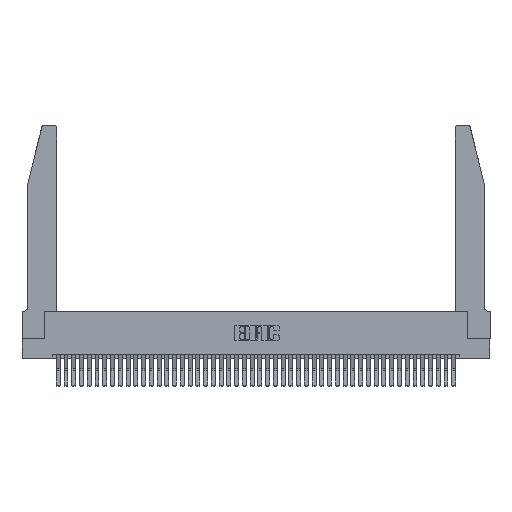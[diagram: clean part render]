
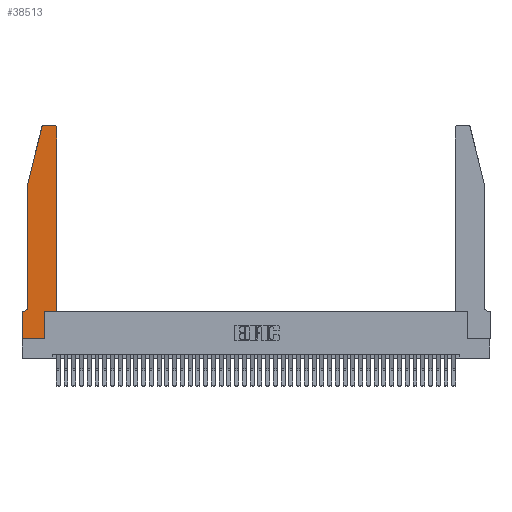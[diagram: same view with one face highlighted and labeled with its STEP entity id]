
A CAD part, top view. The second image highlights one B-rep face of the part: STEP entity #38513.
In plain terms, the highlighted planar face has unit normal (0, 0, 1).
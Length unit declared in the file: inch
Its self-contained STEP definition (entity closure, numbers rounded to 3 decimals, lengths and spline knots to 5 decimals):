
#697 = DIRECTION ( 'NONE',  ( 0., 1., 0. ) ) ;
#743 = VECTOR ( 'NONE', #3688, 39.37008 ) ;
#1118 = VECTOR ( 'NONE', #37977, 39.37008 ) ;
#1593 = CARTESIAN_POINT ( 'NONE',  ( 0., 0., 0.37 ) ) ;
#2560 = EDGE_CURVE ( 'NONE', #4045, #33339, #9989, .T. ) ;
#3688 = DIRECTION ( 'NONE',  ( -1., 0., 0. ) ) ;
#3888 = DIRECTION ( 'NONE',  ( 0., -1., 0. ) ) ;
#4045 = VERTEX_POINT ( 'NONE', #23233 ) ;
#4098 = VERTEX_POINT ( 'NONE', #26815 ) ;
#5146 = CIRCLE ( 'NONE', #24599, 0.03 ) ;
#5670 = CARTESIAN_POINT ( 'NONE',  ( 0.284, 2.72, 0.37 ) ) ;
#6162 = VERTEX_POINT ( 'NONE', #10857 ) ;
#6291 = CARTESIAN_POINT ( 'NONE',  ( 0.0755, 2., 0.37 ) ) ;
#7109 = DIRECTION ( 'NONE',  ( 0., 0., 1. ) ) ;
#8375 = VERTEX_POINT ( 'NONE', #39260 ) ;
#9040 = ORIENTED_EDGE ( 'NONE', *, *, #27470, .T. ) ;
#9112 = DIRECTION ( 'NONE',  ( 1., 0., 0. ) ) ;
#9331 = VERTEX_POINT ( 'NONE', #37391 ) ;
#9704 = DIRECTION ( 'NONE',  ( -0.239, -0.971, 0. ) ) ;
#9774 = ORIENTED_EDGE ( 'NONE', *, *, #19802, .T. ) ;
#9989 = LINE ( 'NONE', #37610, #11072 ) ;
#10232 = EDGE_CURVE ( 'NONE', #9331, #28431, #39793, .T. ) ;
#10234 = DIRECTION ( 'NONE',  ( 0., 0., -1. ) ) ;
#10281 = LINE ( 'NONE', #1593, #27451 ) ;
#10396 = CARTESIAN_POINT ( 'NONE',  ( 0.0755, 0.35, 0.37 ) ) ;
#10463 = EDGE_CURVE ( 'NONE', #4098, #33312, #25434, .T. ) ;
#10784 = CARTESIAN_POINT ( 'NONE',  ( 0.4505, 0.35, 0.37 ) ) ;
#10857 = CARTESIAN_POINT ( 'NONE',  ( 0., 0.35, 0.37 ) ) ;
#11072 = VECTOR ( 'NONE', #17156, 39.37008 ) ;
#11172 = VECTOR ( 'NONE', #25249, 39.37008 ) ;
#11872 = DIRECTION ( 'NONE',  ( 1., 0., 0. ) ) ;
#12148 = CIRCLE ( 'NONE', #27035, 0.07 ) ;
#14380 = AXIS2_PLACEMENT_3D ( 'NONE', #40033, #19575, #43493 ) ;
#14421 = ORIENTED_EDGE ( 'NONE', *, *, #43104, .T. ) ;
#15156 = VECTOR ( 'NONE', #29114, 39.37008 ) ;
#15763 = CARTESIAN_POINT ( 'NONE',  ( 0.2865, 0.35, 0.37 ) ) ;
#16032 = CARTESIAN_POINT ( 'NONE',  ( 0.0755, 2., 0.37 ) ) ;
#17156 = DIRECTION ( 'NONE',  ( -1., 0., 0. ) ) ;
#18472 = CARTESIAN_POINT ( 'NONE',  ( 0.4505, 2.72, 0.37 ) ) ;
#19575 = DIRECTION ( 'NONE',  ( 0., 0., 1. ) ) ;
#19802 = EDGE_CURVE ( 'NONE', #33312, #9331, #38509, .T. ) ;
#20725 = CARTESIAN_POINT ( 'NONE',  ( 0., 0.35, 0.37 ) ) ;
#21437 = VERTEX_POINT ( 'NONE', #16032 ) ;
#22743 = ORIENTED_EDGE ( 'NONE', *, *, #10463, .T. ) ;
#22835 = CARTESIAN_POINT ( 'NONE',  ( 0.25487, 2.72718, 0.37 ) ) ;
#23220 = ORIENTED_EDGE ( 'NONE', *, *, #32648, .T. ) ;
#23233 = CARTESIAN_POINT ( 'NONE',  ( 0.4205, 2.75, 0.37 ) ) ;
#23672 = ORIENTED_EDGE ( 'NONE', *, *, #25031, .T. ) ;
#23761 = EDGE_CURVE ( 'NONE', #27353, #8375, #12148, .T. ) ;
#23864 = VECTOR ( 'NONE', #9704, 39.37008 ) ;
#24190 = ORIENTED_EDGE ( 'NONE', *, *, #30425, .T. ) ;
#24599 = AXIS2_PLACEMENT_3D ( 'NONE', #5670, #29650, #9112 ) ;
#25031 = EDGE_CURVE ( 'NONE', #28431, #4045, #44247, .T. ) ;
#25249 = DIRECTION ( 'NONE',  ( 0., -1., 0. ) ) ;
#25434 = LINE ( 'NONE', #25711, #15156 ) ;
#25711 = CARTESIAN_POINT ( 'NONE',  ( 0.2865, 0.35, 0.37 ) ) ;
#26815 = CARTESIAN_POINT ( 'NONE',  ( 0.2865, 0., 0.37 ) ) ;
#27035 = AXIS2_PLACEMENT_3D ( 'NONE', #30773, #10234, #34166 ) ;
#27353 = VERTEX_POINT ( 'NONE', #28403 ) ;
#27451 = VECTOR ( 'NONE', #11872, 39.37008 ) ;
#27470 = EDGE_CURVE ( 'NONE', #35048, #4098, #10281, .T. ) ;
#27621 = PLANE ( 'NONE',  #42997 ) ;
#28058 = LINE ( 'NONE', #10396, #743 ) ;
#28403 = CARTESIAN_POINT ( 'NONE',  ( 0.0755, 0.42, 0.37 ) ) ;
#28431 = VERTEX_POINT ( 'NONE', #18472 ) ;
#28751 = ORIENTED_EDGE ( 'NONE', *, *, #42319, .T. ) ;
#29114 = DIRECTION ( 'NONE',  ( 0., 1., 0. ) ) ;
#29442 = LINE ( 'NONE', #42246, #11172 ) ;
#29596 = CARTESIAN_POINT ( 'NONE',  ( 0.284, 2.75, 0.37 ) ) ;
#29650 = DIRECTION ( 'NONE',  ( 0., 0., 1. ) ) ;
#30240 = LINE ( 'NONE', #34523, #38187 ) ;
#30425 = EDGE_CURVE ( 'NONE', #6162, #35048, #29442, .T. ) ;
#30502 = EDGE_LOOP ( 'NONE', ( #39063, #23220, #28751, #38084, #43970, #14421, #24190, #9040, #22743, #9774, #37140, #23672 ) ) ;
#30612 = VERTEX_POINT ( 'NONE', #22835 ) ;
#30752 = VECTOR ( 'NONE', #697, 39.37008 ) ;
#30773 = CARTESIAN_POINT ( 'NONE',  ( 0.0055, 0.42, 0.37 ) ) ;
#31051 = DIRECTION ( 'NONE',  ( 1., 0., 0. ) ) ;
#32648 = EDGE_CURVE ( 'NONE', #33339, #30612, #5146, .T. ) ;
#32976 = CARTESIAN_POINT ( 'NONE',  ( 0., 0., 0.37 ) ) ;
#33312 = VERTEX_POINT ( 'NONE', #15763 ) ;
#33339 = VERTEX_POINT ( 'NONE', #29596 ) ;
#34166 = DIRECTION ( 'NONE',  ( -1., 0., 0. ) ) ;
#34523 = CARTESIAN_POINT ( 'NONE',  ( 0.0755, 2., 0.37 ) ) ;
#34753 = CARTESIAN_POINT ( 'NONE',  ( 0.4505, 0.35, 0.37 ) ) ;
#35048 = VERTEX_POINT ( 'NONE', #32976 ) ;
#36564 = FACE_OUTER_BOUND ( 'NONE', #30502, .T. ) ;
#37140 = ORIENTED_EDGE ( 'NONE', *, *, #10232, .T. ) ;
#37391 = CARTESIAN_POINT ( 'NONE',  ( 0.4505, 0.35, 0.37 ) ) ;
#37610 = CARTESIAN_POINT ( 'NONE',  ( 0.2605, 2.75, 0.37 ) ) ;
#37977 = DIRECTION ( 'NONE',  ( 1., 0., 0. ) ) ;
#38084 = ORIENTED_EDGE ( 'NONE', *, *, #42612, .T. ) ;
#38187 = VECTOR ( 'NONE', #3888, 39.37008 ) ;
#38509 = LINE ( 'NONE', #10784, #1118 ) ;
#38513 = ADVANCED_FACE ( 'NONE', ( #36564 ), #27621, .T. ) ;
#39063 = ORIENTED_EDGE ( 'NONE', *, *, #2560, .T. ) ;
#39260 = CARTESIAN_POINT ( 'NONE',  ( 0.0055, 0.35, 0.37 ) ) ;
#39793 = LINE ( 'NONE', #34753, #30752 ) ;
#40033 = CARTESIAN_POINT ( 'NONE',  ( 0.4205, 2.72, 0.37 ) ) ;
#42014 = LINE ( 'NONE', #6291, #23864 ) ;
#42246 = CARTESIAN_POINT ( 'NONE',  ( 0., 0., 0.37 ) ) ;
#42319 = EDGE_CURVE ( 'NONE', #30612, #21437, #42014, .T. ) ;
#42612 = EDGE_CURVE ( 'NONE', #21437, #27353, #30240, .T. ) ;
#42997 = AXIS2_PLACEMENT_3D ( 'NONE', #20725, #7109, #31051 ) ;
#43104 = EDGE_CURVE ( 'NONE', #8375, #6162, #28058, .T. ) ;
#43493 = DIRECTION ( 'NONE',  ( 1., 0., 0. ) ) ;
#43970 = ORIENTED_EDGE ( 'NONE', *, *, #23761, .T. ) ;
#44247 = CIRCLE ( 'NONE', #14380, 0.03 ) ;
